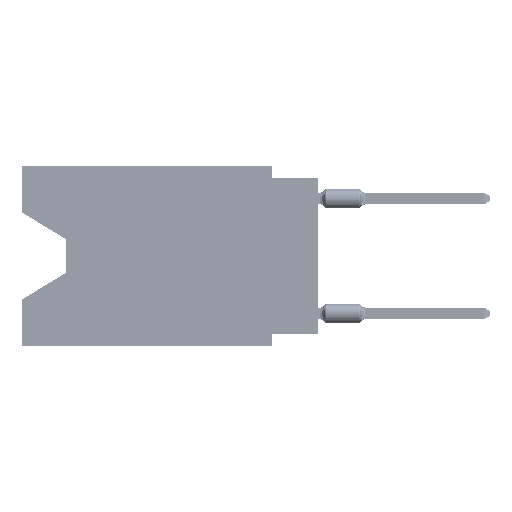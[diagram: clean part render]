
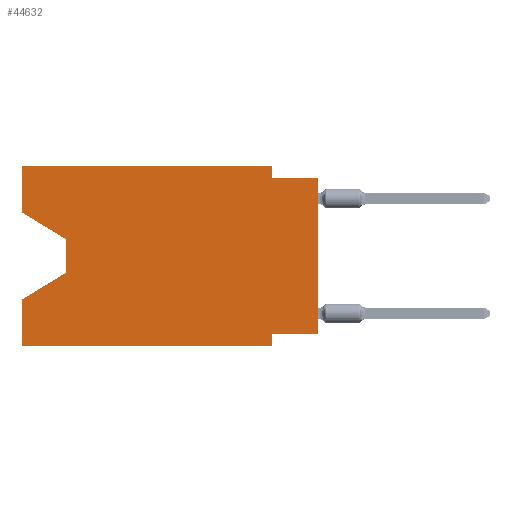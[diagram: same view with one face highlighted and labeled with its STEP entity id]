
A CAD part, left-side view. The second image highlights one B-rep face of the part: STEP entity #44632.
In plain terms, the highlighted planar face has unit normal (-1, 0, 0).
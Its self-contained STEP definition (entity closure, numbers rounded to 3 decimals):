
#956 = ORIENTED_EDGE ( 'NONE', *, *, #67621, .T. ) ;
#959 = EDGE_CURVE ( 'NONE', #43247, #11716, #45523, .T. ) ;
#987 = VERTEX_POINT ( 'NONE', #59856 ) ;
#997 = CARTESIAN_POINT ( 'NONE',  ( 0., 0., 0. ) ) ;
#1264 = LINE ( 'NONE', #57747, #16238 ) ;
#1379 = CARTESIAN_POINT ( 'NONE',  ( 0., 16.383, -9.906 ) ) ;
#4735 = DIRECTION ( 'NONE',  ( 0., 0., 1. ) ) ;
#5561 = LINE ( 'NONE', #1379, #21226 ) ;
#6867 = EDGE_CURVE ( 'NONE', #21935, #987, #1264, .T. ) ;
#7621 = CARTESIAN_POINT ( 'NONE',  ( 0., 16.383, 0. ) ) ;
#8645 = DIRECTION ( 'NONE',  ( 0., 0., 1. ) ) ;
#11716 = VERTEX_POINT ( 'NONE', #30385 ) ;
#11911 = CARTESIAN_POINT ( 'NONE',  ( 0., 0., -0.635 ) ) ;
#13197 = CARTESIAN_POINT ( 'NONE',  ( 0., 16.383, 0. ) ) ;
#13472 = VERTEX_POINT ( 'NONE', #29855 ) ;
#15134 = ORIENTED_EDGE ( 'NONE', *, *, #34569, .T. ) ;
#15289 = DIRECTION ( 'NONE',  ( 0., -1., 0. ) ) ;
#15827 = VERTEX_POINT ( 'NONE', #70077 ) ;
#16238 = VECTOR ( 'NONE', #85126, 1000. ) ;
#17433 = DIRECTION ( 'NONE',  ( 0., -1., 0. ) ) ;
#21226 = VECTOR ( 'NONE', #15289, 1000. ) ;
#21935 = VERTEX_POINT ( 'NONE', #83599 ) ;
#23065 = VECTOR ( 'NONE', #81443, 1000. ) ;
#23945 = ORIENTED_EDGE ( 'NONE', *, *, #80468, .F. ) ;
#24112 = CARTESIAN_POINT ( 'NONE',  ( 0., 2.54, -0.635 ) ) ;
#24921 = ORIENTED_EDGE ( 'NONE', *, *, #68333, .F. ) ;
#24963 = DIRECTION ( 'NONE',  ( 0., 0., -1. ) ) ;
#25671 = VERTEX_POINT ( 'NONE', #11911 ) ;
#26180 = FACE_OUTER_BOUND ( 'NONE', #43097, .T. ) ;
#26522 = LINE ( 'NONE', #88419, #86817 ) ;
#27563 = CARTESIAN_POINT ( 'NONE',  ( 0., 0., -9.271 ) ) ;
#28690 = LINE ( 'NONE', #7621, #31236 ) ;
#28807 = LINE ( 'NONE', #997, #50507 ) ;
#29020 = CARTESIAN_POINT ( 'NONE',  ( 0., 2.54, -9.906 ) ) ;
#29605 = ORIENTED_EDGE ( 'NONE', *, *, #6867, .T. ) ;
#29855 = CARTESIAN_POINT ( 'NONE',  ( 0., 2.54, -9.271 ) ) ;
#29979 = LINE ( 'NONE', #85586, #51162 ) ;
#30364 = CARTESIAN_POINT ( 'NONE',  ( 0., 16.383, -9.906 ) ) ;
#30385 = CARTESIAN_POINT ( 'NONE',  ( 0., 16.383, 0. ) ) ;
#30778 = EDGE_CURVE ( 'NONE', #36057, #21935, #73811, .T. ) ;
#31236 = VECTOR ( 'NONE', #34500, 1000. ) ;
#31250 = CARTESIAN_POINT ( 'NONE',  ( 0., 2.54, 0. ) ) ;
#31678 = EDGE_CURVE ( 'NONE', #13472, #57442, #68645, .T. ) ;
#32311 = VECTOR ( 'NONE', #59173, 1000. ) ;
#34278 = ORIENTED_EDGE ( 'NONE', *, *, #66819, .F. ) ;
#34500 = DIRECTION ( 'NONE',  ( 0., 0., 1. ) ) ;
#34569 = EDGE_CURVE ( 'NONE', #71058, #25671, #28807, .T. ) ;
#34935 = ORIENTED_EDGE ( 'NONE', *, *, #31678, .F. ) ;
#34965 = DIRECTION ( 'NONE',  ( 0., 0., -1. ) ) ;
#35605 = EDGE_CURVE ( 'NONE', #15827, #82752, #65787, .T. ) ;
#36057 = VERTEX_POINT ( 'NONE', #82550 ) ;
#39173 = DIRECTION ( 'NONE',  ( 1., 0., 0. ) ) ;
#39935 = CARTESIAN_POINT ( 'NONE',  ( 0., 2.54, -9.906 ) ) ;
#42703 = VECTOR ( 'NONE', #4735, 1000. ) ;
#43097 = EDGE_LOOP ( 'NONE', ( #956, #48546, #29605, #74114, #64872, #34935, #23945, #15134, #34278, #50648, #24921, #86707 ) ) ;
#43247 = VERTEX_POINT ( 'NONE', #44147 ) ;
#44147 = CARTESIAN_POINT ( 'NONE',  ( 0., 16.383, -2.546 ) ) ;
#44632 = ADVANCED_FACE ( 'NONE', ( #26180 ), #54395, .F. ) ;
#45523 = LINE ( 'NONE', #74660, #42703 ) ;
#46137 = LINE ( 'NONE', #72653, #32311 ) ;
#48546 = ORIENTED_EDGE ( 'NONE', *, *, #30778, .T. ) ;
#50507 = VECTOR ( 'NONE', #8645, 1000. ) ;
#50648 = ORIENTED_EDGE ( 'NONE', *, *, #35605, .F. ) ;
#51162 = VECTOR ( 'NONE', #17433, 1000. ) ;
#51452 = AXIS2_PLACEMENT_3D ( 'NONE', #13197, #39173, #66554 ) ;
#52033 = VECTOR ( 'NONE', #74748, 1000. ) ;
#54395 = PLANE ( 'NONE',  #51452 ) ;
#54972 = LINE ( 'NONE', #87757, #52033 ) ;
#57442 = VERTEX_POINT ( 'NONE', #29020 ) ;
#57747 = CARTESIAN_POINT ( 'NONE',  ( 0., 13.97, -5.893 ) ) ;
#58506 = VERTEX_POINT ( 'NONE', #30364 ) ;
#59173 = DIRECTION ( 'NONE',  ( 0., -1., 0. ) ) ;
#59856 = CARTESIAN_POINT ( 'NONE',  ( 0., 16.383, -7.36 ) ) ;
#63787 = EDGE_CURVE ( 'NONE', #58506, #57442, #5561, .T. ) ;
#64872 = ORIENTED_EDGE ( 'NONE', *, *, #63787, .T. ) ;
#65787 = LINE ( 'NONE', #31250, #85042 ) ;
#66554 = DIRECTION ( 'NONE',  ( 0., 0., -1. ) ) ;
#66819 = EDGE_CURVE ( 'NONE', #82752, #25671, #46137, .T. ) ;
#67621 = EDGE_CURVE ( 'NONE', #43247, #36057, #26522, .T. ) ;
#68333 = EDGE_CURVE ( 'NONE', #11716, #15827, #29979, .T. ) ;
#68645 = LINE ( 'NONE', #39935, #76188 ) ;
#70077 = CARTESIAN_POINT ( 'NONE',  ( 0., 2.54, 0. ) ) ;
#71058 = VERTEX_POINT ( 'NONE', #27563 ) ;
#72040 = EDGE_CURVE ( 'NONE', #58506, #987, #28690, .T. ) ;
#72653 = CARTESIAN_POINT ( 'NONE',  ( 0., 0., -0.635 ) ) ;
#73642 = DIRECTION ( 'NONE',  ( 0., -0.855, -0.519 ) ) ;
#73811 = LINE ( 'NONE', #88151, #23065 ) ;
#74114 = ORIENTED_EDGE ( 'NONE', *, *, #72040, .F. ) ;
#74660 = CARTESIAN_POINT ( 'NONE',  ( 0., 16.383, 0. ) ) ;
#74748 = DIRECTION ( 'NONE',  ( 0., 1., 0. ) ) ;
#76188 = VECTOR ( 'NONE', #34965, 1000. ) ;
#80468 = EDGE_CURVE ( 'NONE', #71058, #13472, #54972, .T. ) ;
#81443 = DIRECTION ( 'NONE',  ( 0., 0., -1. ) ) ;
#82550 = CARTESIAN_POINT ( 'NONE',  ( 0., 13.97, -4.013 ) ) ;
#82752 = VERTEX_POINT ( 'NONE', #24112 ) ;
#83599 = CARTESIAN_POINT ( 'NONE',  ( 0., 13.97, -5.893 ) ) ;
#85042 = VECTOR ( 'NONE', #24963, 1000. ) ;
#85126 = DIRECTION ( 'NONE',  ( 0., 0.855, -0.519 ) ) ;
#85586 = CARTESIAN_POINT ( 'NONE',  ( 0., 16.383, 0. ) ) ;
#86707 = ORIENTED_EDGE ( 'NONE', *, *, #959, .F. ) ;
#86817 = VECTOR ( 'NONE', #73642, 1000. ) ;
#87757 = CARTESIAN_POINT ( 'NONE',  ( 0., 0., -9.271 ) ) ;
#88151 = CARTESIAN_POINT ( 'NONE',  ( 0., 13.97, -4.013 ) ) ;
#88419 = CARTESIAN_POINT ( 'NONE',  ( 0., 16.383, -2.546 ) ) ;
